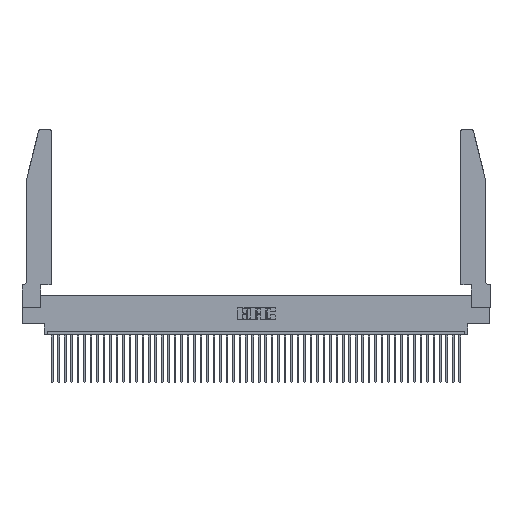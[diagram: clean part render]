
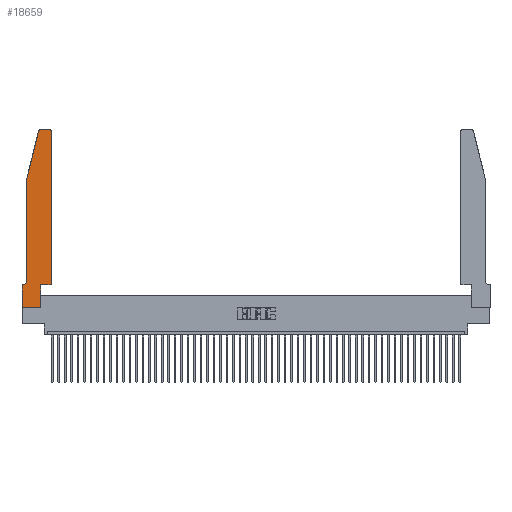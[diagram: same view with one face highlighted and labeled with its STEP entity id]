
A CAD part, top view. The second image highlights one B-rep face of the part: STEP entity #18659.
In plain terms, the highlighted planar face has unit normal (0, 0, 1).
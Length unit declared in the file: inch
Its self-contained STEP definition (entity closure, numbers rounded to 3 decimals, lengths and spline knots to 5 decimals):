
#180 = ORIENTED_EDGE ( 'NONE', *, *, #15858, .T. ) ;
#645 = EDGE_CURVE ( 'NONE', #15625, #29380, #21931, .T. ) ;
#2457 = ORIENTED_EDGE ( 'NONE', *, *, #42135, .T. ) ;
#3191 = DIRECTION ( 'NONE',  ( 1., 0., 0. ) ) ;
#3621 = CARTESIAN_POINT ( 'NONE',  ( 0.4205, 2.72, 0.37 ) ) ;
#4218 = CARTESIAN_POINT ( 'NONE',  ( 0.2865, 0.35, 0.37 ) ) ;
#4395 = VECTOR ( 'NONE', #38529, 39.37008 ) ;
#4983 = AXIS2_PLACEMENT_3D ( 'NONE', #3621, #27472, #15439 ) ;
#5140 = CARTESIAN_POINT ( 'NONE',  ( 0.0755, 2., 0.37 ) ) ;
#5485 = DIRECTION ( 'NONE',  ( 0., -1., 0. ) ) ;
#5524 = CARTESIAN_POINT ( 'NONE',  ( 0.4505, 0.35, 0.37 ) ) ;
#5936 = CIRCLE ( 'NONE', #39802, 0.07 ) ;
#6690 = VERTEX_POINT ( 'NONE', #26433 ) ;
#7034 = EDGE_CURVE ( 'NONE', #48042, #9488, #41752, .T. ) ;
#7150 = CARTESIAN_POINT ( 'NONE',  ( 0.2605, 2.75, 0.37 ) ) ;
#7442 = CARTESIAN_POINT ( 'NONE',  ( 0.284, 2.75, 0.37 ) ) ;
#7621 = ORIENTED_EDGE ( 'NONE', *, *, #15648, .T. ) ;
#7663 = CARTESIAN_POINT ( 'NONE',  ( 0., 0., 0.37 ) ) ;
#8315 = EDGE_CURVE ( 'NONE', #45467, #15625, #5936, .T. ) ;
#8450 = AXIS2_PLACEMENT_3D ( 'NONE', #30745, #49478, #3191 ) ;
#8723 = VERTEX_POINT ( 'NONE', #44449 ) ;
#8774 = CARTESIAN_POINT ( 'NONE',  ( 0.2865, 0., 0.37 ) ) ;
#8856 = DIRECTION ( 'NONE',  ( 1., 0., 0. ) ) ;
#8944 = DIRECTION ( 'NONE',  ( -0.239, -0.971, 0. ) ) ;
#9488 = VERTEX_POINT ( 'NONE', #7442 ) ;
#9643 = CIRCLE ( 'NONE', #4983, 0.03 ) ;
#9679 = LINE ( 'NONE', #28233, #41180 ) ;
#10070 = EDGE_CURVE ( 'NONE', #29380, #6690, #15363, .T. ) ;
#10626 = ORIENTED_EDGE ( 'NONE', *, *, #42181, .T. ) ;
#11441 = VERTEX_POINT ( 'NONE', #8774 ) ;
#11451 = ORIENTED_EDGE ( 'NONE', *, *, #19325, .T. ) ;
#12131 = CARTESIAN_POINT ( 'NONE',  ( 0., 0.35, 0.37 ) ) ;
#12194 = VERTEX_POINT ( 'NONE', #49696 ) ;
#13180 = VECTOR ( 'NONE', #35596, 39.37008 ) ;
#13814 = CARTESIAN_POINT ( 'NONE',  ( 0.0755, 0.42, 0.37 ) ) ;
#15102 = CARTESIAN_POINT ( 'NONE',  ( 0.4205, 2.75, 0.37 ) ) ;
#15363 = LINE ( 'NONE', #31673, #37747 ) ;
#15439 = DIRECTION ( 'NONE',  ( 1., 0., 0. ) ) ;
#15508 = VECTOR ( 'NONE', #5485, 39.37008 ) ;
#15625 = VERTEX_POINT ( 'NONE', #25435 ) ;
#15648 = EDGE_CURVE ( 'NONE', #6690, #11441, #23161, .T. ) ;
#15858 = EDGE_CURVE ( 'NONE', #17853, #8723, #28524, .T. ) ;
#16124 = DIRECTION ( 'NONE',  ( 0., 0., 1. ) ) ;
#16579 = DIRECTION ( 'NONE',  ( 1., 0., 0. ) ) ;
#17486 = ORIENTED_EDGE ( 'NONE', *, *, #44525, .T. ) ;
#17853 = VERTEX_POINT ( 'NONE', #39918 ) ;
#18659 = ADVANCED_FACE ( 'NONE', ( #21268 ), #32006, .T. ) ;
#19171 = DIRECTION ( 'NONE',  ( 0., 0., -1. ) ) ;
#19325 = EDGE_CURVE ( 'NONE', #40562, #12194, #9679, .T. ) ;
#21201 = VECTOR ( 'NONE', #34194, 39.37008 ) ;
#21268 = FACE_OUTER_BOUND ( 'NONE', #40201, .T. ) ;
#21931 = LINE ( 'NONE', #45922, #4395 ) ;
#23161 = LINE ( 'NONE', #7663, #40083 ) ;
#23886 = VECTOR ( 'NONE', #27374, 39.37008 ) ;
#25435 = CARTESIAN_POINT ( 'NONE',  ( 0.0055, 0.35, 0.37 ) ) ;
#25688 = LINE ( 'NONE', #4218, #23886 ) ;
#26433 = CARTESIAN_POINT ( 'NONE',  ( 0., 0., 0.37 ) ) ;
#27374 = DIRECTION ( 'NONE',  ( 0., 1., 0. ) ) ;
#27472 = DIRECTION ( 'NONE',  ( 0., 0., 1. ) ) ;
#28074 = CIRCLE ( 'NONE', #8450, 0.03 ) ;
#28233 = CARTESIAN_POINT ( 'NONE',  ( 0.0755, 2., 0.37 ) ) ;
#28524 = LINE ( 'NONE', #38599, #43065 ) ;
#29380 = VERTEX_POINT ( 'NONE', #12131 ) ;
#30745 = CARTESIAN_POINT ( 'NONE',  ( 0.284, 2.72, 0.37 ) ) ;
#30869 = ORIENTED_EDGE ( 'NONE', *, *, #10070, .T. ) ;
#31056 = CARTESIAN_POINT ( 'NONE',  ( 0.0055, 0.42, 0.37 ) ) ;
#31496 = EDGE_CURVE ( 'NONE', #12194, #45467, #47552, .T. ) ;
#31635 = VERTEX_POINT ( 'NONE', #44660 ) ;
#31673 = CARTESIAN_POINT ( 'NONE',  ( 0., 0., 0.37 ) ) ;
#32006 = PLANE ( 'NONE',  #36981 ) ;
#34194 = DIRECTION ( 'NONE',  ( -1., 0., 0. ) ) ;
#34854 = ORIENTED_EDGE ( 'NONE', *, *, #49660, .T. ) ;
#35596 = DIRECTION ( 'NONE',  ( 1., 0., 0. ) ) ;
#35733 = CARTESIAN_POINT ( 'NONE',  ( 0., 0.35, 0.37 ) ) ;
#36232 = DIRECTION ( 'NONE',  ( 0., -1., 0. ) ) ;
#36822 = LINE ( 'NONE', #5524, #13180 ) ;
#36981 = AXIS2_PLACEMENT_3D ( 'NONE', #35733, #16124, #8856 ) ;
#37747 = VECTOR ( 'NONE', #36232, 39.37008 ) ;
#38191 = CARTESIAN_POINT ( 'NONE',  ( 0.25487, 2.72718, 0.37 ) ) ;
#38529 = DIRECTION ( 'NONE',  ( -1., 0., 0. ) ) ;
#38599 = CARTESIAN_POINT ( 'NONE',  ( 0.4505, 0.35, 0.37 ) ) ;
#39802 = AXIS2_PLACEMENT_3D ( 'NONE', #31056, #19171, #46546 ) ;
#39918 = CARTESIAN_POINT ( 'NONE',  ( 0.4505, 0.35, 0.37 ) ) ;
#40083 = VECTOR ( 'NONE', #16579, 39.37008 ) ;
#40201 = EDGE_LOOP ( 'NONE', ( #43465, #2457, #11451, #49074, #42493, #43512, #30869, #7621, #10626, #34854, #180, #17486 ) ) ;
#40562 = VERTEX_POINT ( 'NONE', #38191 ) ;
#41180 = VECTOR ( 'NONE', #8944, 39.37008 ) ;
#41752 = LINE ( 'NONE', #7150, #21201 ) ;
#42135 = EDGE_CURVE ( 'NONE', #9488, #40562, #28074, .T. ) ;
#42181 = EDGE_CURVE ( 'NONE', #11441, #31635, #25688, .T. ) ;
#42493 = ORIENTED_EDGE ( 'NONE', *, *, #8315, .T. ) ;
#43065 = VECTOR ( 'NONE', #46330, 39.37008 ) ;
#43465 = ORIENTED_EDGE ( 'NONE', *, *, #7034, .T. ) ;
#43512 = ORIENTED_EDGE ( 'NONE', *, *, #645, .T. ) ;
#44449 = CARTESIAN_POINT ( 'NONE',  ( 0.4505, 2.72, 0.37 ) ) ;
#44525 = EDGE_CURVE ( 'NONE', #8723, #48042, #9643, .T. ) ;
#44660 = CARTESIAN_POINT ( 'NONE',  ( 0.2865, 0.35, 0.37 ) ) ;
#45467 = VERTEX_POINT ( 'NONE', #13814 ) ;
#45922 = CARTESIAN_POINT ( 'NONE',  ( 0.0755, 0.35, 0.37 ) ) ;
#46330 = DIRECTION ( 'NONE',  ( 0., 1., 0. ) ) ;
#46546 = DIRECTION ( 'NONE',  ( -1., 0., 0. ) ) ;
#47552 = LINE ( 'NONE', #5140, #15508 ) ;
#48042 = VERTEX_POINT ( 'NONE', #15102 ) ;
#49074 = ORIENTED_EDGE ( 'NONE', *, *, #31496, .T. ) ;
#49478 = DIRECTION ( 'NONE',  ( 0., 0., 1. ) ) ;
#49660 = EDGE_CURVE ( 'NONE', #31635, #17853, #36822, .T. ) ;
#49696 = CARTESIAN_POINT ( 'NONE',  ( 0.0755, 2., 0.37 ) ) ;
